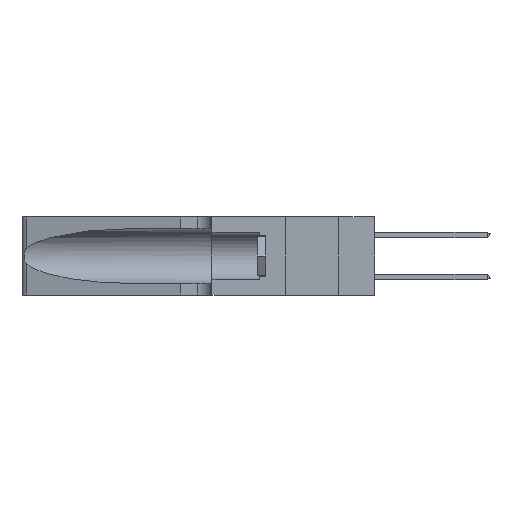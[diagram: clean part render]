
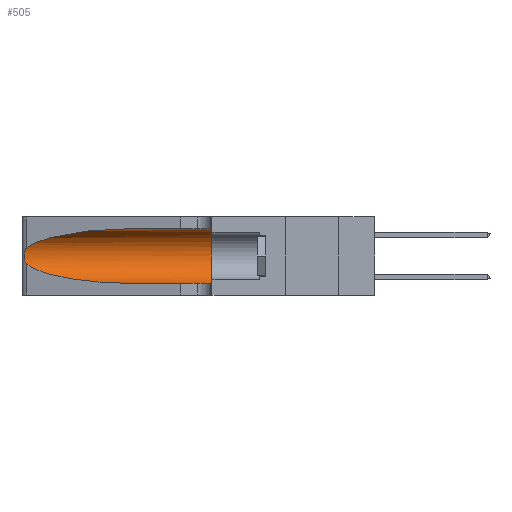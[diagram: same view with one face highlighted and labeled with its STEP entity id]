
A CAD part, left-side view. The second image highlights one B-rep face of the part: STEP entity #505.
In plain terms, the highlighted cylindrical face has radius 3.308 mm (diameter 6.617 mm), a partial arc.
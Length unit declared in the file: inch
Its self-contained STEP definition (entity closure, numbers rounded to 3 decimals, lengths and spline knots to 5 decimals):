
#229 = EDGE_CURVE ( 'NONE', #13565, #13172, #8108, .T. ) ;
#480 = CARTESIAN_POINT ( 'NONE',  ( 0.25854, 1.2359, 0.20912 ) ) ;
#505 = ADVANCED_FACE ( 'NONE', ( #3196 ), #21793, .F. ) ;
#949 = DIRECTION ( 'NONE',  ( 0., -1., 0. ) ) ;
#1761 = CARTESIAN_POINT ( 'NONE',  ( 0.1305, 0.35, 0.185 ) ) ;
#2358 = CARTESIAN_POINT ( 'NONE',  ( 0.1305, 0.35, 0.31525 ) ) ;
#2518 = CARTESIAN_POINT ( 'NONE',  ( 0.26075, 1.23896, 0.19203 ) ) ;
#2687 = EDGE_CURVE ( 'NONE', #13913, #13172, #16687, .T. ) ;
#2928 = CARTESIAN_POINT ( 'NONE',  ( 0.1305, 1.61858, 0.31525 ) ) ;
#3196 = FACE_OUTER_BOUND ( 'NONE', #16545, .T. ) ;
#4425 = CARTESIAN_POINT ( 'NONE',  ( 0.25555, 1.22994, 0.2215 ) ) ;
#4516 = CARTESIAN_POINT ( 'NONE',  ( 0.26017, 1.23833, 0.17102 ) ) ;
#4928 = DIRECTION ( 'NONE',  ( 0., -1., 0. ) ) ;
#4970 =( BOUNDED_CURVE ( )  B_SPLINE_CURVE ( 3, ( #16663, #14843, #16748, #5220 ),
 .UNSPECIFIED., .F., .T. ) 
 B_SPLINE_CURVE_WITH_KNOTS ( ( 4, 4 ),
 ( 3.44316, 4.71239 ),
 .UNSPECIFIED. ) 
 CURVE ( )  GEOMETRIC_REPRESENTATION_ITEM ( )  RATIONAL_B_SPLINE_CURVE ( ( 1., 0.87, 0.87, 1. ) ) 
 REPRESENTATION_ITEM ( '' )  );
#5116 = CARTESIAN_POINT ( 'NONE',  ( 0.1305, 0.72297, 0.05475 ) ) ;
#5220 = CARTESIAN_POINT ( 'NONE',  ( 0.1305, 0.72297, 0.05475 ) ) ;
#5316 = ORIENTED_EDGE ( 'NONE', *, *, #21163, .F. ) ;
#5404 = VERTEX_POINT ( 'NONE', #18317 ) ;
#6493 = CARTESIAN_POINT ( 'NONE',  ( 0.25789, 1.23486, 0.15765 ) ) ;
#8108 = CIRCLE ( 'NONE', #11927, 0.13025 ) ;
#8412 = EDGE_CURVE ( 'NONE', #19515, #9903, #8693, .T. ) ;
#8421 = CARTESIAN_POINT ( 'NONE',  ( 0.25555, 1.22993, 0.14849 ) ) ;
#8693 = B_SPLINE_CURVE_WITH_KNOTS ( 'NONE', 3,
 ( #10289, #4425, #15990, #12236, #480, #14163, #2518, #16075, #4516, #17958, #6493, #19844, #8421, #21733 ),
 .UNSPECIFIED., .F., .F.,
 ( 4, 2, 2, 2, 2, 2, 4 ),
 ( 0., 0.00027, 0.00053, 0.00107, 0.0016, 0.00187, 0.00214 ),
 .UNSPECIFIED. ) ;
#8730 = CARTESIAN_POINT ( 'NONE',  ( 0.25487, 1.22718, 0.22369 ) ) ;
#8955 = DIRECTION ( 'NONE',  ( 0., 0., -1. ) ) ;
#9149 = CARTESIAN_POINT ( 'NONE',  ( 0.25487, 1.22718, 0.14631 ) ) ;
#9476 =( BOUNDED_CURVE ( )  B_SPLINE_CURVE ( 3, ( #16363, #18263, #20141, #8730 ),
 .UNSPECIFIED., .F., .F. ) 
 B_SPLINE_CURVE_WITH_KNOTS ( ( 4, 4 ),
 ( 1.5708, 2.84003 ),
 .UNSPECIFIED. ) 
 CURVE ( )  GEOMETRIC_REPRESENTATION_ITEM ( )  RATIONAL_B_SPLINE_CURVE ( ( 1., 0.87, 0.87, 1. ) ) 
 REPRESENTATION_ITEM ( '' )  );
#9903 = VERTEX_POINT ( 'NONE', #9149 ) ;
#10289 = CARTESIAN_POINT ( 'NONE',  ( 0.25487, 1.22718, 0.22369 ) ) ;
#10443 = ORIENTED_EDGE ( 'NONE', *, *, #8412, .T. ) ;
#10900 = CARTESIAN_POINT ( 'NONE',  ( 0.1305, 0.35, 0.05475 ) ) ;
#11609 = VECTOR ( 'NONE', #949, 39.37008 ) ;
#11927 = AXIS2_PLACEMENT_3D ( 'NONE', #1761, #18886, #14054 ) ;
#12236 = CARTESIAN_POINT ( 'NONE',  ( 0.25787, 1.23484, 0.2124 ) ) ;
#12588 = ORIENTED_EDGE ( 'NONE', *, *, #229, .F. ) ;
#12812 = CARTESIAN_POINT ( 'NONE',  ( 0.1305, 1.61858, 0.185 ) ) ;
#13172 = VERTEX_POINT ( 'NONE', #10900 ) ;
#13565 = VERTEX_POINT ( 'NONE', #2358 ) ;
#13913 = VERTEX_POINT ( 'NONE', #5116 ) ;
#14054 = DIRECTION ( 'NONE',  ( 0., 0., 1. ) ) ;
#14163 = CARTESIAN_POINT ( 'NONE',  ( 0.26018, 1.23835, 0.19895 ) ) ;
#14843 = CARTESIAN_POINT ( 'NONE',  ( 0.2373, 1.15595, 0.08982 ) ) ;
#15990 = CARTESIAN_POINT ( 'NONE',  ( 0.25639, 1.23184, 0.21858 ) ) ;
#16075 = CARTESIAN_POINT ( 'NONE',  ( 0.26075, 1.23896, 0.178 ) ) ;
#16363 = CARTESIAN_POINT ( 'NONE',  ( 0.1305, 0.72297, 0.31525 ) ) ;
#16545 = EDGE_LOOP ( 'NONE', ( #22586, #10443, #22882, #24653, #12588, #5316 ) ) ;
#16560 = AXIS2_PLACEMENT_3D ( 'NONE', #12812, #21244, #8955 ) ;
#16663 = CARTESIAN_POINT ( 'NONE',  ( 0.25487, 1.22718, 0.14631 ) ) ;
#16687 = LINE ( 'NONE', #21465, #11609 ) ;
#16748 = CARTESIAN_POINT ( 'NONE',  ( 0.18966, 0.96281, 0.05475 ) ) ;
#17372 = VECTOR ( 'NONE', #4928, 39.37008 ) ;
#17958 = CARTESIAN_POINT ( 'NONE',  ( 0.25856, 1.23593, 0.16098 ) ) ;
#18263 = CARTESIAN_POINT ( 'NONE',  ( 0.18966, 0.96281, 0.31525 ) ) ;
#18317 = CARTESIAN_POINT ( 'NONE',  ( 0.1305, 0.72297, 0.31525 ) ) ;
#18886 = DIRECTION ( 'NONE',  ( 0., 1., 0. ) ) ;
#19515 = VERTEX_POINT ( 'NONE', #24550 ) ;
#19844 = CARTESIAN_POINT ( 'NONE',  ( 0.25639, 1.23186, 0.15144 ) ) ;
#20141 = CARTESIAN_POINT ( 'NONE',  ( 0.2373, 1.15595, 0.28018 ) ) ;
#21163 = EDGE_CURVE ( 'NONE', #5404, #13565, #22354, .T. ) ;
#21244 = DIRECTION ( 'NONE',  ( 0., -1., 0. ) ) ;
#21465 = CARTESIAN_POINT ( 'NONE',  ( 0.1305, 1.61858, 0.05475 ) ) ;
#21733 = CARTESIAN_POINT ( 'NONE',  ( 0.25487, 1.22718, 0.14631 ) ) ;
#21793 = CYLINDRICAL_SURFACE ( 'NONE', #16560, 0.13025 ) ;
#22354 = LINE ( 'NONE', #2928, #17372 ) ;
#22586 = ORIENTED_EDGE ( 'NONE', *, *, #23451, .T. ) ;
#22882 = ORIENTED_EDGE ( 'NONE', *, *, #24235, .T. ) ;
#23451 = EDGE_CURVE ( 'NONE', #5404, #19515, #9476, .T. ) ;
#24235 = EDGE_CURVE ( 'NONE', #9903, #13913, #4970, .T. ) ;
#24550 = CARTESIAN_POINT ( 'NONE',  ( 0.25487, 1.22718, 0.22369 ) ) ;
#24653 = ORIENTED_EDGE ( 'NONE', *, *, #2687, .T. ) ;
